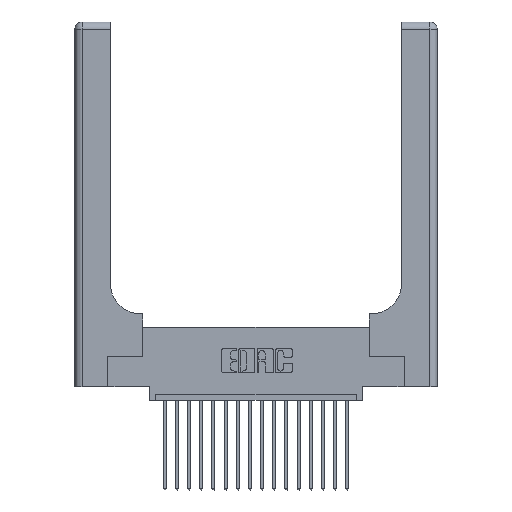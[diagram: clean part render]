
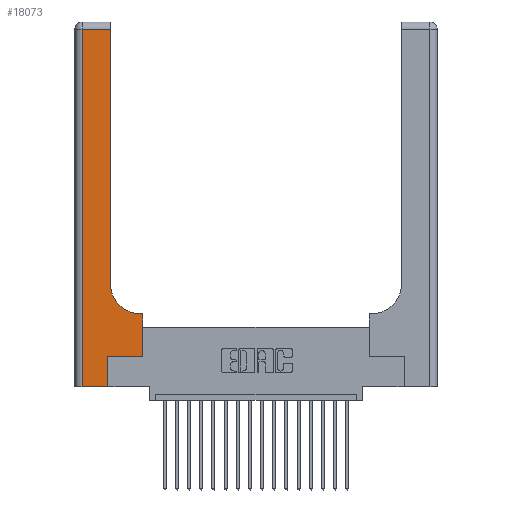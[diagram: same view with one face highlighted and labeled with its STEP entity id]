
A CAD part, top view. The second image highlights one B-rep face of the part: STEP entity #18073.
In plain terms, the highlighted planar face has unit normal (0, 0, 1).
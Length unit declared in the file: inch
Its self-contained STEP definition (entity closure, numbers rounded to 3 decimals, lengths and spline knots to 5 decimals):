
#920 = CARTESIAN_POINT ( 'NONE',  ( 0.5585, 0.25, 0.37 ) ) ;
#953 = VECTOR ( 'NONE', #20122, 39.37008 ) ;
#1078 = EDGE_CURVE ( 'NONE', #5346, #13489, #4433, .T. ) ;
#1343 = CARTESIAN_POINT ( 'NONE',  ( 0.06, 3., 0.37 ) ) ;
#1369 = DIRECTION ( 'NONE',  ( 1., 0., 0. ) ) ;
#1438 = EDGE_CURVE ( 'NONE', #7563, #5346, #20065, .T. ) ;
#1756 = EDGE_CURVE ( 'NONE', #15223, #14930, #18004, .T. ) ;
#2303 = VECTOR ( 'NONE', #1369, 39.37008 ) ;
#2666 = CARTESIAN_POINT ( 'NONE',  ( 0.2915, 2.94, 0.37 ) ) ;
#2739 = CARTESIAN_POINT ( 'NONE',  ( 0.2915, 0.6, 0.37 ) ) ;
#2783 = ORIENTED_EDGE ( 'NONE', *, *, #5581, .T. ) ;
#2964 = DIRECTION ( 'NONE',  ( -1., 0., 0. ) ) ;
#3675 = DIRECTION ( 'NONE',  ( -1., 0., 0. ) ) ;
#3747 = LINE ( 'NONE', #9712, #953 ) ;
#4297 = CARTESIAN_POINT ( 'NONE',  ( 0.269, 0., 0.37 ) ) ;
#4433 = LINE ( 'NONE', #13866, #7449 ) ;
#4444 = VECTOR ( 'NONE', #17432, 39.37008 ) ;
#4493 = CARTESIAN_POINT ( 'NONE',  ( 0.06, 2.94, 0.37 ) ) ;
#5204 = CARTESIAN_POINT ( 'NONE',  ( 0.269, 0.25, 0.37 ) ) ;
#5346 = VERTEX_POINT ( 'NONE', #19462 ) ;
#5350 = PLANE ( 'NONE',  #6233 ) ;
#5456 = LINE ( 'NONE', #19402, #13324 ) ;
#5581 = EDGE_CURVE ( 'NONE', #13489, #18733, #3747, .T. ) ;
#5764 = ORIENTED_EDGE ( 'NONE', *, *, #12182, .T. ) ;
#5962 = ORIENTED_EDGE ( 'NONE', *, *, #10728, .T. ) ;
#6158 = CARTESIAN_POINT ( 'NONE',  ( 0.5415, 0.6, 0.37 ) ) ;
#6233 = AXIS2_PLACEMENT_3D ( 'NONE', #8604, #18235, #3675 ) ;
#6378 = ORIENTED_EDGE ( 'NONE', *, *, #6597, .T. ) ;
#6597 = EDGE_CURVE ( 'NONE', #14930, #7563, #14311, .T. ) ;
#6907 = ORIENTED_EDGE ( 'NONE', *, *, #17828, .T. ) ;
#7440 = LINE ( 'NONE', #1343, #4444 ) ;
#7449 = VECTOR ( 'NONE', #12231, 39.37008 ) ;
#7563 = VERTEX_POINT ( 'NONE', #6158 ) ;
#8210 = DIRECTION ( 'NONE',  ( 0., 1., 0. ) ) ;
#8343 = DIRECTION ( 'NONE',  ( 0., 1., 0. ) ) ;
#8604 = CARTESIAN_POINT ( 'NONE',  ( 0., 3., 0.37 ) ) ;
#9414 = EDGE_LOOP ( 'NONE', ( #19234, #2783, #5764, #5962, #13502, #6907, #15109, #6378, #10570 ) ) ;
#9432 = CARTESIAN_POINT ( 'NONE',  ( 0.06, 0., 0.37 ) ) ;
#9631 = DIRECTION ( 'NONE',  ( 0., 0., -1. ) ) ;
#9693 = EDGE_CURVE ( 'NONE', #10057, #17377, #18864, .T. ) ;
#9712 = CARTESIAN_POINT ( 'NONE',  ( 0., 2.94, 0.37 ) ) ;
#10057 = VERTEX_POINT ( 'NONE', #4297 ) ;
#10135 = FACE_OUTER_BOUND ( 'NONE', #9414, .T. ) ;
#10570 = ORIENTED_EDGE ( 'NONE', *, *, #1438, .T. ) ;
#10585 = VECTOR ( 'NONE', #8343, 39.37008 ) ;
#10728 = EDGE_CURVE ( 'NONE', #18348, #10057, #5456, .T. ) ;
#11078 = AXIS2_PLACEMENT_3D ( 'NONE', #17530, #9631, #16071 ) ;
#11382 = DIRECTION ( 'NONE',  ( 1., 0., 0. ) ) ;
#12182 = EDGE_CURVE ( 'NONE', #18733, #18348, #7440, .T. ) ;
#12231 = DIRECTION ( 'NONE',  ( 0., 1., 0. ) ) ;
#13324 = VECTOR ( 'NONE', #11382, 39.37008 ) ;
#13489 = VERTEX_POINT ( 'NONE', #2666 ) ;
#13502 = ORIENTED_EDGE ( 'NONE', *, *, #9693, .T. ) ;
#13508 = VECTOR ( 'NONE', #8210, 39.37008 ) ;
#13866 = CARTESIAN_POINT ( 'NONE',  ( 0.2915, 3., 0.37 ) ) ;
#13942 = CARTESIAN_POINT ( 'NONE',  ( 0.5585, 0.6, 0.37 ) ) ;
#14311 = LINE ( 'NONE', #2739, #14804 ) ;
#14688 = LINE ( 'NONE', #20699, #2303 ) ;
#14804 = VECTOR ( 'NONE', #2964, 39.37008 ) ;
#14930 = VERTEX_POINT ( 'NONE', #13942 ) ;
#15109 = ORIENTED_EDGE ( 'NONE', *, *, #1756, .T. ) ;
#15223 = VERTEX_POINT ( 'NONE', #920 ) ;
#16071 = DIRECTION ( 'NONE',  ( 1., 0., 0. ) ) ;
#16270 = CARTESIAN_POINT ( 'NONE',  ( 0.5585, 0.25, 0.37 ) ) ;
#17377 = VERTEX_POINT ( 'NONE', #5204 ) ;
#17432 = DIRECTION ( 'NONE',  ( 0., -1., 0. ) ) ;
#17530 = CARTESIAN_POINT ( 'NONE',  ( 0.5415, 0.85, 0.37 ) ) ;
#17828 = EDGE_CURVE ( 'NONE', #17377, #15223, #14688, .T. ) ;
#17848 = CARTESIAN_POINT ( 'NONE',  ( 0.269, 0., 0.37 ) ) ;
#18004 = LINE ( 'NONE', #16270, #13508 ) ;
#18073 = ADVANCED_FACE ( 'NONE', ( #10135 ), #5350, .F. ) ;
#18235 = DIRECTION ( 'NONE',  ( 0., 0., -1. ) ) ;
#18348 = VERTEX_POINT ( 'NONE', #9432 ) ;
#18733 = VERTEX_POINT ( 'NONE', #4493 ) ;
#18864 = LINE ( 'NONE', #17848, #10585 ) ;
#19234 = ORIENTED_EDGE ( 'NONE', *, *, #1078, .T. ) ;
#19402 = CARTESIAN_POINT ( 'NONE',  ( 0., 0., 0.37 ) ) ;
#19462 = CARTESIAN_POINT ( 'NONE',  ( 0.2915, 0.85, 0.37 ) ) ;
#20065 = CIRCLE ( 'NONE', #11078, 0.25 ) ;
#20122 = DIRECTION ( 'NONE',  ( -1., 0., 0. ) ) ;
#20699 = CARTESIAN_POINT ( 'NONE',  ( 0.269, 0.25, 0.37 ) ) ;
